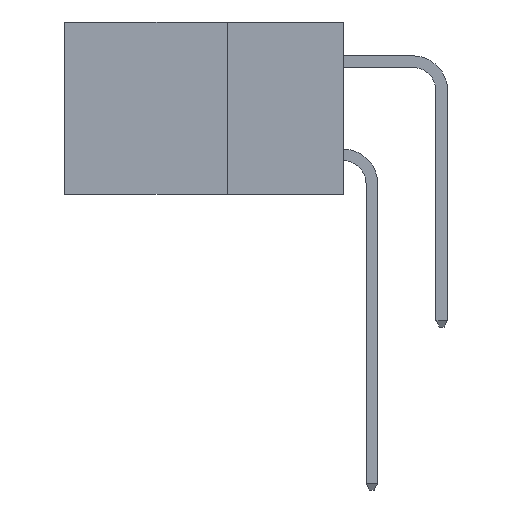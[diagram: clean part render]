
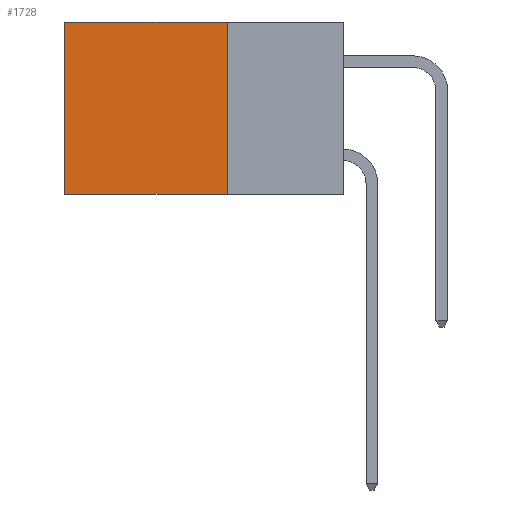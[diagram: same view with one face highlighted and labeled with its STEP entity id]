
A CAD part, left-side view. The second image highlights one B-rep face of the part: STEP entity #1728.
In plain terms, the highlighted planar face has unit normal (-1, 0, 0).
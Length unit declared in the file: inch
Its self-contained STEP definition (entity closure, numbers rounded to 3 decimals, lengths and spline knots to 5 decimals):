
#1629 = CARTESIAN_POINT ( 'NONE',  ( 0.2615, 0.6, -0.37 ) ) ;
#1728 = ADVANCED_FACE ( 'NONE', ( #13160 ), #4595, .F. ) ;
#2259 = EDGE_CURVE ( 'NONE', #3786, #3599, #5483, .T. ) ;
#2680 = CARTESIAN_POINT ( 'NONE',  ( 0.2615, 0.25, -0.37 ) ) ;
#3188 = DIRECTION ( 'NONE',  ( 0., 1., 0. ) ) ;
#3258 = ORIENTED_EDGE ( 'NONE', *, *, #2259, .T. ) ;
#3341 = CARTESIAN_POINT ( 'NONE',  ( 0.2615, 0.25, 0. ) ) ;
#3599 = VERTEX_POINT ( 'NONE', #11503 ) ;
#3786 = VERTEX_POINT ( 'NONE', #13790 ) ;
#4115 = VERTEX_POINT ( 'NONE', #12302 ) ;
#4388 = VECTOR ( 'NONE', #11963, 39.37008 ) ;
#4595 = PLANE ( 'NONE',  #14818 ) ;
#4710 = CARTESIAN_POINT ( 'NONE',  ( 0.2615, 0.25, -0.37 ) ) ;
#4938 = DIRECTION ( 'NONE',  ( 1., 0., 0. ) ) ;
#5483 = LINE ( 'NONE', #3341, #8544 ) ;
#7086 = EDGE_CURVE ( 'NONE', #3599, #7935, #8406, .T. ) ;
#7162 = VECTOR ( 'NONE', #8405, 39.37008 ) ;
#7458 = LINE ( 'NONE', #11985, #4388 ) ;
#7466 = DIRECTION ( 'NONE',  ( 0., 0., -1. ) ) ;
#7935 = VERTEX_POINT ( 'NONE', #1629 ) ;
#8405 = DIRECTION ( 'NONE',  ( 0., 0., -1. ) ) ;
#8406 = LINE ( 'NONE', #9082, #14256 ) ;
#8544 = VECTOR ( 'NONE', #3188, 39.37008 ) ;
#9002 = DIRECTION ( 'NONE',  ( 0., 0., -1. ) ) ;
#9082 = CARTESIAN_POINT ( 'NONE',  ( 0.2615, 0.6, -0.37 ) ) ;
#9310 = EDGE_CURVE ( 'NONE', #4115, #7935, #7458, .T. ) ;
#10149 = ORIENTED_EDGE ( 'NONE', *, *, #13320, .F. ) ;
#11503 = CARTESIAN_POINT ( 'NONE',  ( 0.2615, 0.6, 0. ) ) ;
#11963 = DIRECTION ( 'NONE',  ( 0., 1., 0. ) ) ;
#11985 = CARTESIAN_POINT ( 'NONE',  ( 0.2615, 0.25, -0.37 ) ) ;
#12302 = CARTESIAN_POINT ( 'NONE',  ( 0.2615, 0.25, -0.37 ) ) ;
#12478 = EDGE_LOOP ( 'NONE', ( #14607, #14571, #10149, #3258 ) ) ;
#12656 = LINE ( 'NONE', #2680, #7162 ) ;
#13160 = FACE_OUTER_BOUND ( 'NONE', #12478, .T. ) ;
#13320 = EDGE_CURVE ( 'NONE', #3786, #4115, #12656, .T. ) ;
#13790 = CARTESIAN_POINT ( 'NONE',  ( 0.2615, 0.25, 0. ) ) ;
#14256 = VECTOR ( 'NONE', #9002, 39.37008 ) ;
#14571 = ORIENTED_EDGE ( 'NONE', *, *, #9310, .F. ) ;
#14607 = ORIENTED_EDGE ( 'NONE', *, *, #7086, .T. ) ;
#14818 = AXIS2_PLACEMENT_3D ( 'NONE', #4710, #4938, #7466 ) ;
